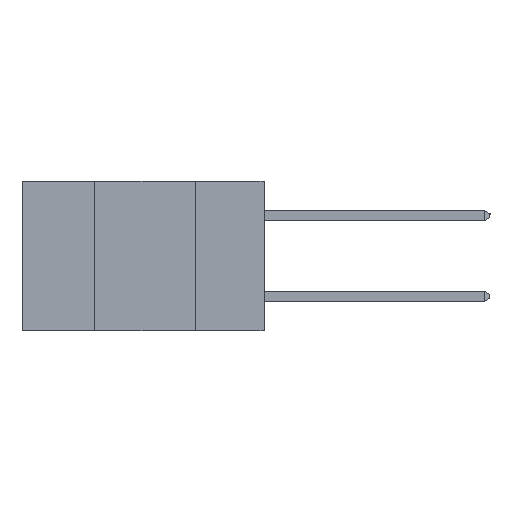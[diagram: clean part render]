
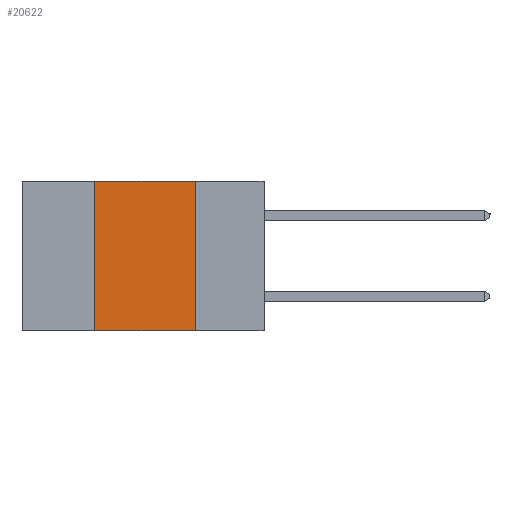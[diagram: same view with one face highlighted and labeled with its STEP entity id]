
A CAD part, left-side view. The second image highlights one B-rep face of the part: STEP entity #20622.
In plain terms, the highlighted planar face has unit normal (-1, 0, 0).
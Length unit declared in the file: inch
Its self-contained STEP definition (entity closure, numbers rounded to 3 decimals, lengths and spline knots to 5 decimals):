
#491 = EDGE_CURVE ( 'NONE', #9146, #11579, #4694, .T. ) ;
#646 = DIRECTION ( 'NONE',  ( 1., 0., 0. ) ) ;
#782 = CARTESIAN_POINT ( 'NONE',  ( 0., 0.6, 0. ) ) ;
#1059 = DIRECTION ( 'NONE',  ( 0., -1., 0. ) ) ;
#2173 = DIRECTION ( 'NONE',  ( 0., 0., -1. ) ) ;
#2279 = CARTESIAN_POINT ( 'NONE',  ( 0., 0.17, 0. ) ) ;
#2905 = VECTOR ( 'NONE', #16392, 39.37008 ) ;
#3344 = VERTEX_POINT ( 'NONE', #13474 ) ;
#3610 = LINE ( 'NONE', #7829, #2905 ) ;
#4694 = LINE ( 'NONE', #6389, #12078 ) ;
#5343 = ORIENTED_EDGE ( 'NONE', *, *, #491, .F. ) ;
#5970 = CARTESIAN_POINT ( 'NONE',  ( 0., 0.42, -0.37 ) ) ;
#6389 = CARTESIAN_POINT ( 'NONE',  ( 0., 0.17, -0.37 ) ) ;
#6432 = EDGE_CURVE ( 'NONE', #3344, #11579, #3610, .T. ) ;
#6806 = ORIENTED_EDGE ( 'NONE', *, *, #6432, .T. ) ;
#7159 = CARTESIAN_POINT ( 'NONE',  ( 0., 0.17, -0.37 ) ) ;
#7829 = CARTESIAN_POINT ( 'NONE',  ( 0., 0.6, -0.37 ) ) ;
#7939 = LINE ( 'NONE', #5970, #20062 ) ;
#8211 = AXIS2_PLACEMENT_3D ( 'NONE', #13554, #646, #21702 ) ;
#9146 = VERTEX_POINT ( 'NONE', #2279 ) ;
#10783 = EDGE_CURVE ( 'NONE', #3344, #16383, #7939, .T. ) ;
#11579 = VERTEX_POINT ( 'NONE', #7159 ) ;
#12078 = VECTOR ( 'NONE', #2173, 39.37008 ) ;
#13474 = CARTESIAN_POINT ( 'NONE',  ( 0., 0.42, -0.37 ) ) ;
#13554 = CARTESIAN_POINT ( 'NONE',  ( 0., 0.6, 0. ) ) ;
#13629 = ORIENTED_EDGE ( 'NONE', *, *, #10783, .F. ) ;
#14156 = VECTOR ( 'NONE', #1059, 39.37008 ) ;
#15847 = CARTESIAN_POINT ( 'NONE',  ( 0., 0.42, 0. ) ) ;
#16383 = VERTEX_POINT ( 'NONE', #15847 ) ;
#16392 = DIRECTION ( 'NONE',  ( 0., -1., 0. ) ) ;
#17238 = EDGE_LOOP ( 'NONE', ( #5343, #25982, #13629, #6806 ) ) ;
#17364 = PLANE ( 'NONE',  #8211 ) ;
#20031 = LINE ( 'NONE', #782, #14156 ) ;
#20062 = VECTOR ( 'NONE', #20845, 39.37008 ) ;
#20622 = ADVANCED_FACE ( 'NONE', ( #23814 ), #17364, .F. ) ;
#20845 = DIRECTION ( 'NONE',  ( 0., 0., 1. ) ) ;
#21702 = DIRECTION ( 'NONE',  ( 0., 0., -1. ) ) ;
#23814 = FACE_OUTER_BOUND ( 'NONE', #17238, .T. ) ;
#23837 = EDGE_CURVE ( 'NONE', #16383, #9146, #20031, .T. ) ;
#25982 = ORIENTED_EDGE ( 'NONE', *, *, #23837, .F. ) ;
